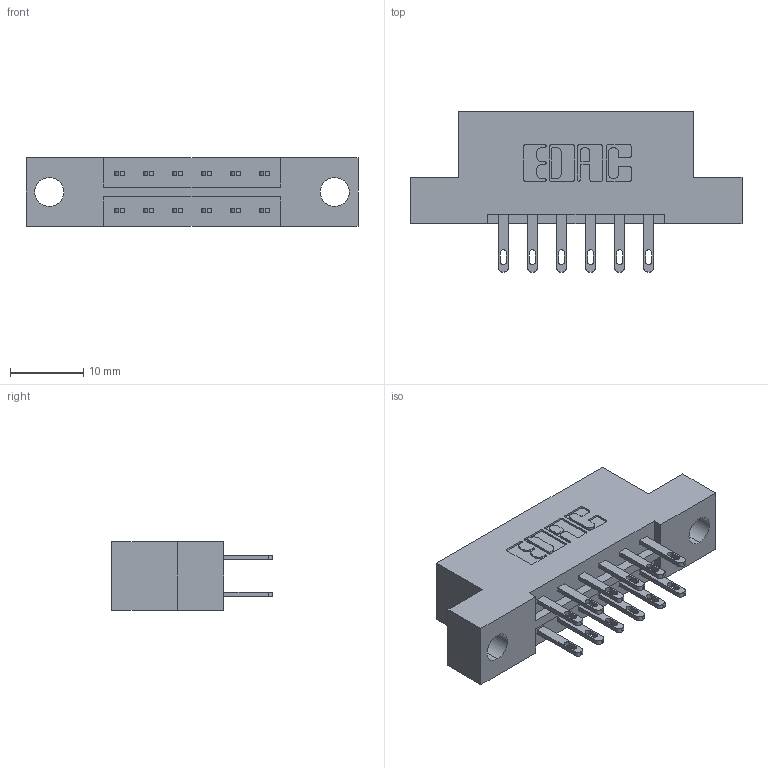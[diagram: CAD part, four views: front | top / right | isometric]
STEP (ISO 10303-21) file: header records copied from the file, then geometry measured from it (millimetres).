
FILE_DESCRIPTION (( 'STEP AP203' ), '1' );
FILE_NAME ('333-012-500-204.STEP', '2018-07-31T23:47:41', ( '' ), ( '' ), 'SwSTEP 2.0', 'SolidWorks 2016', '' );
FILE_SCHEMA (( 'CONFIG_CONTROL_DESIGN' ));
Length unit declared in the file: inch
Products named in the file (3): 345-292-001_345-293-100; 333-012-500-204; 333 Part_Flush - .156 Dia - TH
Assembly tree (13 placements, depth 2):
  333-012-500-204
    333 Part_Flush - .156 Dia - TH
    345-292-001_345-293-100  x12
Bounding box: 45.31 x 21.85 x 9.4 mm (x, y, z)
Volume: 4238.4 mm3; surface area: 4555.5 mm2
Topology: 13 solids, 13 shells, 690 faces, 2075 edges, 1382 vertices
Faces by surface type: plane 430, cylinder 260
Entity records: 8449 total; most frequent: CARTESIAN_POINT 1442, ORIENTED_EDGE 1378, DIRECTION 1297, EDGE_CURVE 689, VECTOR 557, LINE 557, VERTEX_POINT 458, AXIS2_PLACEMENT_3D 370
